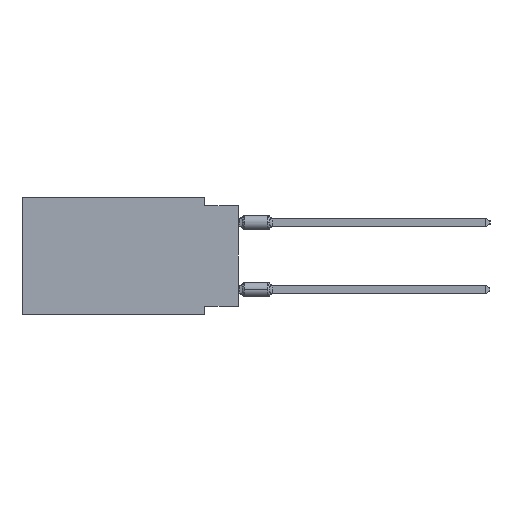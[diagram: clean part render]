
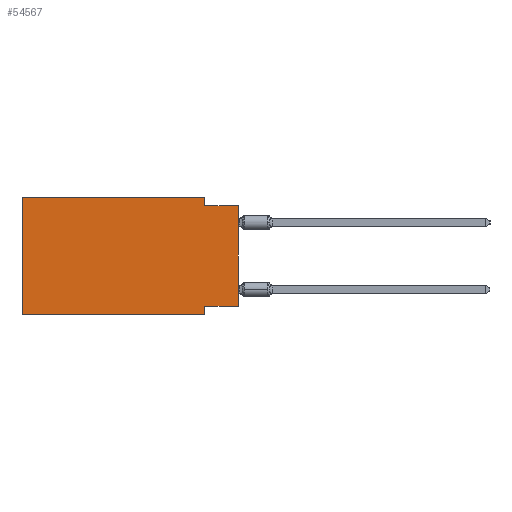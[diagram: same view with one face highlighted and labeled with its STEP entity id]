
A CAD part, left-side view. The second image highlights one B-rep face of the part: STEP entity #54567.
In plain terms, the highlighted planar face has unit normal (-1, 0, 0).
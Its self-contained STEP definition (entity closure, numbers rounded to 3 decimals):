
#744 = ORIENTED_EDGE ( 'NONE', *, *, #43050, .F. ) ;
#800 = EDGE_CURVE ( 'NONE', #9222, #32672, #28738, .T. ) ;
#1211 = ORIENTED_EDGE ( 'NONE', *, *, #20987, .F. ) ;
#1680 = LINE ( 'NONE', #23346, #49511 ) ;
#2784 = ORIENTED_EDGE ( 'NONE', *, *, #38652, .T. ) ;
#3056 = VERTEX_POINT ( 'NONE', #45919 ) ;
#3506 = EDGE_CURVE ( 'NONE', #12295, #19656, #45850, .T. ) ;
#6230 = DIRECTION ( 'NONE',  ( 0., -1., 0. ) ) ;
#6317 = CARTESIAN_POINT ( 'NONE',  ( 0., 2.54, 0. ) ) ;
#6385 = PLANE ( 'NONE',  #44266 ) ;
#6697 = CARTESIAN_POINT ( 'NONE',  ( 0., 2.54, 0. ) ) ;
#7711 = VECTOR ( 'NONE', #27394, 1000. ) ;
#8236 = EDGE_LOOP ( 'NONE', ( #55541, #55710, #18669, #1211, #25178, #2784, #41958, #744 ) ) ;
#9222 = VERTEX_POINT ( 'NONE', #18172 ) ;
#10233 = EDGE_CURVE ( 'NONE', #15861, #33642, #44464, .T. ) ;
#10590 = DIRECTION ( 'NONE',  ( 0., -1., 0. ) ) ;
#11357 = CARTESIAN_POINT ( 'NONE',  ( 0., 16.383, 0. ) ) ;
#11498 = FACE_OUTER_BOUND ( 'NONE', #8236, .T. ) ;
#12295 = VERTEX_POINT ( 'NONE', #25523 ) ;
#14862 = CARTESIAN_POINT ( 'NONE',  ( 0., 0., -0.635 ) ) ;
#15861 = VERTEX_POINT ( 'NONE', #55858 ) ;
#17751 = CARTESIAN_POINT ( 'NONE',  ( 0., 0., -8.255 ) ) ;
#17952 = VECTOR ( 'NONE', #10590, 1000. ) ;
#18172 = CARTESIAN_POINT ( 'NONE',  ( 0., 16.383, -8.89 ) ) ;
#18586 = CARTESIAN_POINT ( 'NONE',  ( 0., 2.54, -8.89 ) ) ;
#18669 = ORIENTED_EDGE ( 'NONE', *, *, #54946, .F. ) ;
#18895 = VERTEX_POINT ( 'NONE', #6697 ) ;
#19656 = VERTEX_POINT ( 'NONE', #47305 ) ;
#20987 = EDGE_CURVE ( 'NONE', #32672, #18895, #30644, .T. ) ;
#21172 = DIRECTION ( 'NONE',  ( 0., 1., 0. ) ) ;
#23346 = CARTESIAN_POINT ( 'NONE',  ( 0., 16.383, -8.89 ) ) ;
#23421 = DIRECTION ( 'NONE',  ( 0., 0., -1. ) ) ;
#24604 = DIRECTION ( 'NONE',  ( 1., 0., 0. ) ) ;
#24848 = CARTESIAN_POINT ( 'NONE',  ( 0., 16.383, 0. ) ) ;
#25178 = ORIENTED_EDGE ( 'NONE', *, *, #800, .F. ) ;
#25523 = CARTESIAN_POINT ( 'NONE',  ( 0., 0., -8.255 ) ) ;
#26292 = LINE ( 'NONE', #17751, #38517 ) ;
#27394 = DIRECTION ( 'NONE',  ( 0., 0., -1. ) ) ;
#28738 = LINE ( 'NONE', #11357, #33504 ) ;
#30372 = DIRECTION ( 'NONE',  ( 0., -1., 0. ) ) ;
#30644 = LINE ( 'NONE', #39191, #43964 ) ;
#32672 = VERTEX_POINT ( 'NONE', #24848 ) ;
#32717 = DIRECTION ( 'NONE',  ( 0., 0., 1. ) ) ;
#33504 = VECTOR ( 'NONE', #32717, 1000. ) ;
#33642 = VERTEX_POINT ( 'NONE', #44035 ) ;
#36498 = LINE ( 'NONE', #6317, #41576 ) ;
#37610 = CARTESIAN_POINT ( 'NONE',  ( 0., 0., 0. ) ) ;
#38517 = VECTOR ( 'NONE', #21172, 1000. ) ;
#38652 = EDGE_CURVE ( 'NONE', #9222, #33642, #1680, .T. ) ;
#39191 = CARTESIAN_POINT ( 'NONE',  ( 0., 16.383, 0. ) ) ;
#41576 = VECTOR ( 'NONE', #23421, 1000. ) ;
#41883 = LINE ( 'NONE', #14862, #17952 ) ;
#41958 = ORIENTED_EDGE ( 'NONE', *, *, #10233, .F. ) ;
#43050 = EDGE_CURVE ( 'NONE', #12295, #15861, #26292, .T. ) ;
#43964 = VECTOR ( 'NONE', #30372, 1000. ) ;
#44035 = CARTESIAN_POINT ( 'NONE',  ( 0., 2.54, -8.89 ) ) ;
#44266 = AXIS2_PLACEMENT_3D ( 'NONE', #46202, #24604, #50209 ) ;
#44464 = LINE ( 'NONE', #18586, #7711 ) ;
#45850 = LINE ( 'NONE', #37610, #56292 ) ;
#45919 = CARTESIAN_POINT ( 'NONE',  ( 0., 2.54, -0.635 ) ) ;
#46202 = CARTESIAN_POINT ( 'NONE',  ( 0., 16.383, 0. ) ) ;
#47305 = CARTESIAN_POINT ( 'NONE',  ( 0., 0., -0.635 ) ) ;
#49511 = VECTOR ( 'NONE', #6230, 1000. ) ;
#50209 = DIRECTION ( 'NONE',  ( 0., 0., -1. ) ) ;
#54567 = ADVANCED_FACE ( 'NONE', ( #11498 ), #6385, .F. ) ;
#54936 = EDGE_CURVE ( 'NONE', #3056, #19656, #41883, .T. ) ;
#54946 = EDGE_CURVE ( 'NONE', #18895, #3056, #36498, .T. ) ;
#54960 = DIRECTION ( 'NONE',  ( 0., 0., 1. ) ) ;
#55541 = ORIENTED_EDGE ( 'NONE', *, *, #3506, .T. ) ;
#55710 = ORIENTED_EDGE ( 'NONE', *, *, #54936, .F. ) ;
#55858 = CARTESIAN_POINT ( 'NONE',  ( 0., 2.54, -8.255 ) ) ;
#56292 = VECTOR ( 'NONE', #54960, 1000. ) ;
